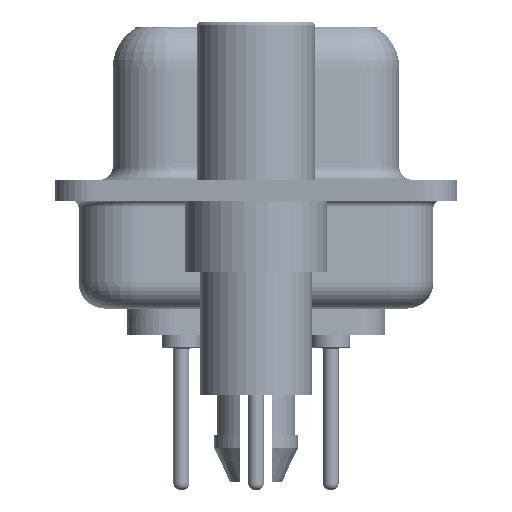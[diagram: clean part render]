
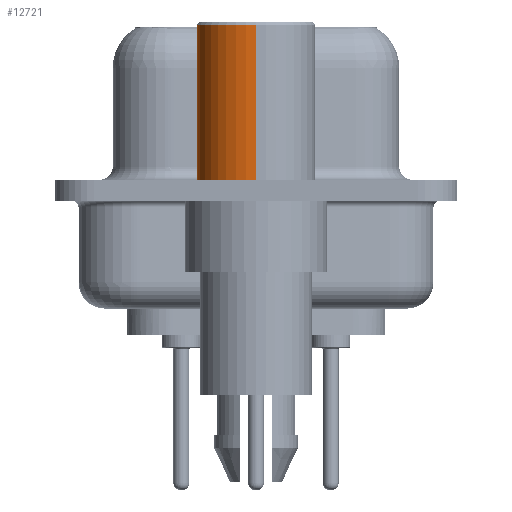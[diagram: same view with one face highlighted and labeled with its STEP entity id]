
A CAD part, left-side view. The second image highlights one B-rep face of the part: STEP entity #12721.
In plain terms, the highlighted cylindrical face has radius 2.25 mm (diameter 4.5 mm), a partial arc.
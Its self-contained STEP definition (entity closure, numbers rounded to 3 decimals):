
#944 = VERTEX_POINT ( 'NONE', #19204 ) ;
#1475 = VECTOR ( 'NONE', #10020, 1000. ) ;
#1985 = CARTESIAN_POINT ( 'NONE',  ( -2.25, 0., 6.3 ) ) ;
#2330 = DIRECTION ( 'NONE',  ( 1., 0., 0. ) ) ;
#2404 = CARTESIAN_POINT ( 'NONE',  ( -2.25, 0., 0.581 ) ) ;
#2688 = VERTEX_POINT ( 'NONE', #14346 ) ;
#3658 = VERTEX_POINT ( 'NONE', #11664 ) ;
#3928 = ORIENTED_EDGE ( 'NONE', *, *, #32975, .F. ) ;
#4623 = CYLINDRICAL_SURFACE ( 'NONE', #29691, 2.25 ) ;
#5502 = EDGE_CURVE ( 'NONE', #3658, #16953, #25600, .T. ) ;
#5611 = DIRECTION ( 'NONE',  ( 0., 0., 1. ) ) ;
#7069 = LINE ( 'NONE', #12899, #21615 ) ;
#8888 = CIRCLE ( 'NONE', #13177, 2.25 ) ;
#10020 = DIRECTION ( 'NONE',  ( 0., 0., 1. ) ) ;
#10845 = DIRECTION ( 'NONE',  ( 1., 0., 0. ) ) ;
#11664 = CARTESIAN_POINT ( 'NONE',  ( -2.25, 0., 0.4 ) ) ;
#12017 = ORIENTED_EDGE ( 'NONE', *, *, #5502, .T. ) ;
#12721 = ADVANCED_FACE ( 'NONE', ( #14594 ), #4623, .T. ) ;
#12899 = CARTESIAN_POINT ( 'NONE',  ( 2.25, 0., 0.581 ) ) ;
#13177 = AXIS2_PLACEMENT_3D ( 'NONE', #29117, #5611, #10845 ) ;
#14346 = CARTESIAN_POINT ( 'NONE',  ( 2.25, 0., 0.4 ) ) ;
#14594 = FACE_OUTER_BOUND ( 'NONE', #16083, .T. ) ;
#14705 = AXIS2_PLACEMENT_3D ( 'NONE', #22822, #20580, #2330 ) ;
#14773 = DIRECTION ( 'NONE',  ( 1., 0., 0. ) ) ;
#16083 = EDGE_LOOP ( 'NONE', ( #26457, #12017, #3928, #24937 ) ) ;
#16112 = EDGE_CURVE ( 'NONE', #2688, #944, #7069, .T. ) ;
#16953 = VERTEX_POINT ( 'NONE', #1985 ) ;
#19204 = CARTESIAN_POINT ( 'NONE',  ( 2.25, 0., 6.3 ) ) ;
#20580 = DIRECTION ( 'NONE',  ( 0., 0., 1. ) ) ;
#21615 = VECTOR ( 'NONE', #27523, 1000. ) ;
#22301 = EDGE_CURVE ( 'NONE', #2688, #3658, #8888, .T. ) ;
#22822 = CARTESIAN_POINT ( 'NONE',  ( 0., 0., 6.3 ) ) ;
#24937 = ORIENTED_EDGE ( 'NONE', *, *, #16112, .F. ) ;
#25600 = LINE ( 'NONE', #2404, #1475 ) ;
#26457 = ORIENTED_EDGE ( 'NONE', *, *, #22301, .T. ) ;
#27523 = DIRECTION ( 'NONE',  ( 0., 0., 1. ) ) ;
#27822 = DIRECTION ( 'NONE',  ( 0., 0., 1. ) ) ;
#29117 = CARTESIAN_POINT ( 'NONE',  ( 0., 0., 0.4 ) ) ;
#29691 = AXIS2_PLACEMENT_3D ( 'NONE', #33037, #27822, #14773 ) ;
#30930 = CIRCLE ( 'NONE', #14705, 2.25 ) ;
#32975 = EDGE_CURVE ( 'NONE', #944, #16953, #30930, .T. ) ;
#33037 = CARTESIAN_POINT ( 'NONE',  ( 0., 0., 0.581 ) ) ;
